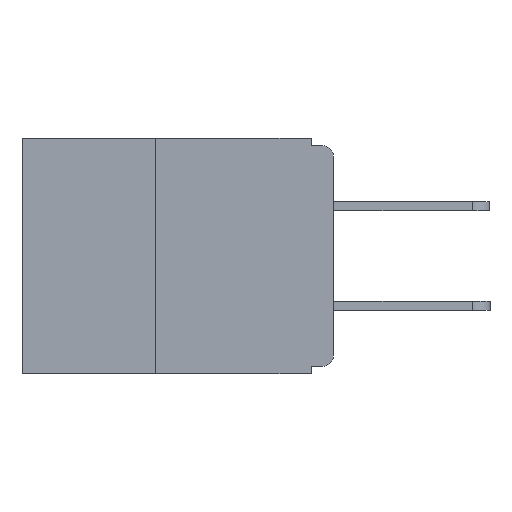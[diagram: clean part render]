
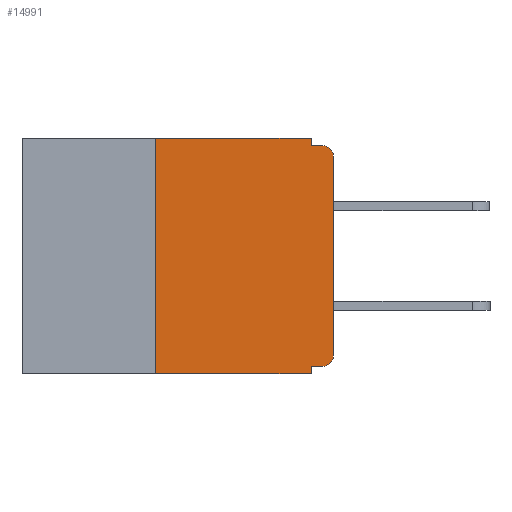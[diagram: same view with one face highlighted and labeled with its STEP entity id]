
A CAD part, left-side view. The second image highlights one B-rep face of the part: STEP entity #14991.
In plain terms, the highlighted planar face has unit normal (-1, 0, 0).
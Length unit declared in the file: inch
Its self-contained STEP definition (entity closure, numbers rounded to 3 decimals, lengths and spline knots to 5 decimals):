
#689 = EDGE_CURVE ( 'NONE', #10929, #18240, #13156, .T. ) ;
#1224 = ORIENTED_EDGE ( 'NONE', *, *, #1648, .T. ) ;
#1319 = VECTOR ( 'NONE', #18168, 39.37008 ) ;
#1648 = EDGE_CURVE ( 'NONE', #3766, #10929, #18512, .T. ) ;
#1651 = VERTEX_POINT ( 'NONE', #11548 ) ;
#1682 = CARTESIAN_POINT ( 'NONE',  ( 0., 0.437, 0. ) ) ;
#1854 = LINE ( 'NONE', #6882, #1319 ) ;
#2036 = AXIS2_PLACEMENT_3D ( 'NONE', #1682, #13304, #3448 ) ;
#2048 = VERTEX_POINT ( 'NONE', #11087 ) ;
#2058 = ORIENTED_EDGE ( 'NONE', *, *, #689, .T. ) ;
#2074 = VERTEX_POINT ( 'NONE', #14423 ) ;
#2195 = ORIENTED_EDGE ( 'NONE', *, *, #13700, .F. ) ;
#2402 = ORIENTED_EDGE ( 'NONE', *, *, #15662, .F. ) ;
#2676 = ORIENTED_EDGE ( 'NONE', *, *, #15551, .F. ) ;
#2717 = ORIENTED_EDGE ( 'NONE', *, *, #18271, .F. ) ;
#2983 = ORIENTED_EDGE ( 'NONE', *, *, #4641, .T. ) ;
#3044 = CARTESIAN_POINT ( 'NONE',  ( 0., 0.031, -0.33 ) ) ;
#3118 = ORIENTED_EDGE ( 'NONE', *, *, #19626, .F. ) ;
#3270 = LINE ( 'NONE', #19368, #19438 ) ;
#3318 = ORIENTED_EDGE ( 'NONE', *, *, #16900, .F. ) ;
#3448 = DIRECTION ( 'NONE',  ( 0., 0., -1. ) ) ;
#3461 = ORIENTED_EDGE ( 'NONE', *, *, #10120, .T. ) ;
#3472 = CARTESIAN_POINT ( 'NONE',  ( 0., 0., -0.01 ) ) ;
#3557 = EDGE_LOOP ( 'NONE', ( #1224, #2058, #2195, #2402, #2676, #2717, #2983, #3118, #3318, #3461 ) ) ;
#3573 = LINE ( 'NONE', #3044, #11807 ) ;
#3690 = VECTOR ( 'NONE', #17099, 39.37008 ) ;
#3766 = VERTEX_POINT ( 'NONE', #10801 ) ;
#4450 = CIRCLE ( 'NONE', #8788, 0.015 ) ;
#4641 = EDGE_CURVE ( 'NONE', #2048, #16286, #9387, .T. ) ;
#5120 = DIRECTION ( 'NONE',  ( 0., -1., 0. ) ) ;
#5570 = VECTOR ( 'NONE', #18267, 39.37008 ) ;
#5923 = CARTESIAN_POINT ( 'NONE',  ( 0., 0.015, -0.32 ) ) ;
#5950 = VECTOR ( 'NONE', #5120, 39.37008 ) ;
#6232 = CARTESIAN_POINT ( 'NONE',  ( 0., 0.015, -0.025 ) ) ;
#6348 = DIRECTION ( 'NONE',  ( 0., 0., -1. ) ) ;
#6848 = DIRECTION ( 'NONE',  ( -1., 0., 0. ) ) ;
#6882 = CARTESIAN_POINT ( 'NONE',  ( 0., 0., -0.32 ) ) ;
#8160 = DIRECTION ( 'NONE',  ( 0., -1., 0. ) ) ;
#8504 = CARTESIAN_POINT ( 'NONE',  ( 0., 0.031, -0.33 ) ) ;
#8788 = AXIS2_PLACEMENT_3D ( 'NONE', #18756, #9176, #20324 ) ;
#9176 = DIRECTION ( 'NONE',  ( -1., 0., 0. ) ) ;
#9387 = LINE ( 'NONE', #18901, #5570 ) ;
#9427 = VERTEX_POINT ( 'NONE', #5923 ) ;
#9596 = DIRECTION ( 'NONE',  ( 0., 0., -1. ) ) ;
#10120 = EDGE_CURVE ( 'NONE', #9427, #3766, #4450, .T. ) ;
#10128 = DIRECTION ( 'NONE',  ( 0., 0., -1. ) ) ;
#10534 = CARTESIAN_POINT ( 'NONE',  ( 0., 0.25, 0. ) ) ;
#10801 = CARTESIAN_POINT ( 'NONE',  ( 0., 0., -0.305 ) ) ;
#10929 = VERTEX_POINT ( 'NONE', #14597 ) ;
#11087 = CARTESIAN_POINT ( 'NONE',  ( 0., 0.25, -0.33 ) ) ;
#11232 = CARTESIAN_POINT ( 'NONE',  ( 0., 0., 0. ) ) ;
#11358 = CARTESIAN_POINT ( 'NONE',  ( 0., 0.031, 0. ) ) ;
#11548 = CARTESIAN_POINT ( 'NONE',  ( 0., 0.031, -0.01 ) ) ;
#11710 = AXIS2_PLACEMENT_3D ( 'NONE', #6232, #6848, #6348 ) ;
#11807 = VECTOR ( 'NONE', #9596, 39.37008 ) ;
#12461 = DIRECTION ( 'NONE',  ( 0., 0., 1. ) ) ;
#13156 = CIRCLE ( 'NONE', #11710, 0.015 ) ;
#13304 = DIRECTION ( 'NONE',  ( 1., 0., 0. ) ) ;
#13305 = VECTOR ( 'NONE', #10128, 39.37008 ) ;
#13371 = VECTOR ( 'NONE', #12461, 39.37008 ) ;
#13416 = CARTESIAN_POINT ( 'NONE',  ( 0., 0.031, 0. ) ) ;
#13700 = EDGE_CURVE ( 'NONE', #1651, #18240, #14653, .T. ) ;
#13830 = LINE ( 'NONE', #13416, #13305 ) ;
#14423 = CARTESIAN_POINT ( 'NONE',  ( 0., 0.031, -0.32 ) ) ;
#14597 = CARTESIAN_POINT ( 'NONE',  ( 0., 0., -0.025 ) ) ;
#14653 = LINE ( 'NONE', #3472, #5950 ) ;
#14991 = ADVANCED_FACE ( 'NONE', ( #20192 ), #16410, .F. ) ;
#15490 = CARTESIAN_POINT ( 'NONE',  ( 0., 0.015, -0.01 ) ) ;
#15551 = EDGE_CURVE ( 'NONE', #19967, #16725, #3270, .T. ) ;
#15561 = CARTESIAN_POINT ( 'NONE',  ( 0., 0.25, -0.33 ) ) ;
#15662 = EDGE_CURVE ( 'NONE', #16725, #1651, #13830, .T. ) ;
#16286 = VERTEX_POINT ( 'NONE', #8504 ) ;
#16410 = PLANE ( 'NONE',  #2036 ) ;
#16725 = VERTEX_POINT ( 'NONE', #11358 ) ;
#16900 = EDGE_CURVE ( 'NONE', #9427, #2074, #1854, .T. ) ;
#17099 = DIRECTION ( 'NONE',  ( 0., 0., 1. ) ) ;
#18168 = DIRECTION ( 'NONE',  ( 0., 1., 0. ) ) ;
#18240 = VERTEX_POINT ( 'NONE', #15490 ) ;
#18267 = DIRECTION ( 'NONE',  ( 0., -1., 0. ) ) ;
#18271 = EDGE_CURVE ( 'NONE', #2048, #19967, #20796, .T. ) ;
#18512 = LINE ( 'NONE', #11232, #13371 ) ;
#18756 = CARTESIAN_POINT ( 'NONE',  ( 0., 0.015, -0.305 ) ) ;
#18901 = CARTESIAN_POINT ( 'NONE',  ( 0., 0.437, -0.33 ) ) ;
#19368 = CARTESIAN_POINT ( 'NONE',  ( 0., 0.437, 0. ) ) ;
#19438 = VECTOR ( 'NONE', #8160, 39.37008 ) ;
#19626 = EDGE_CURVE ( 'NONE', #2074, #16286, #3573, .T. ) ;
#19967 = VERTEX_POINT ( 'NONE', #10534 ) ;
#20192 = FACE_OUTER_BOUND ( 'NONE', #3557, .T. ) ;
#20324 = DIRECTION ( 'NONE',  ( 0., 0., -1. ) ) ;
#20796 = LINE ( 'NONE', #15561, #3690 ) ;
